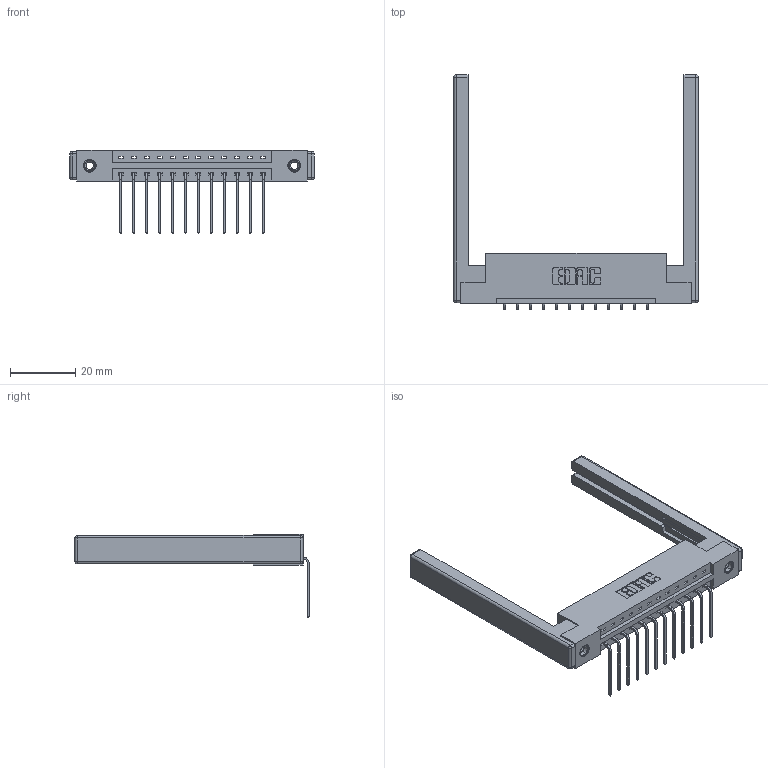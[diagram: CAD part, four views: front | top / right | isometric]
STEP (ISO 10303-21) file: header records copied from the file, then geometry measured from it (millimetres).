
FILE_DESCRIPTION (( 'STEP AP203' ), '1' );
FILE_NAME ('337-012-559-168.STEP', '2019-09-28T01:02:09', ( '' ), ( '' ), 'SwSTEP 2.0', 'SolidWorks 2016', '' );
FILE_SCHEMA (( 'CONFIG_CONTROL_DESIGN' ));
Length unit declared in the file: inch
Products named in the file (5): 345-250-001_345-250-001-102; 337 Part_Flush Mounting Lugs - 0.156 Dia-TI; 345-292-001_558 559 Tail - 1; 307-220-068; 337-012-559-168
Assembly tree (17 placements, depth 2):
  337-012-559-168
    337 Part_Flush Mounting Lugs - 0.156 Dia-TI
    345-292-001_558 559 Tail - 1  x12
    345-250-001_345-250-001-102  x2
    307-220-068  x2
Bounding box: 74.98 x 71.82 x 25.53 mm (x, y, z)
Volume: 11848.8 mm3; surface area: 11878.1 mm2
Topology: 17 solids, 17 shells, 1036 faces, 3029 edges, 1982 vertices
Faces by surface type: plane 734, cylinder 278, cone 12, sphere 8, torus 4
Entity records: 15644 total; most frequent: CARTESIAN_POINT 2679, ORIENTED_EDGE 2616, DIRECTION 2390, EDGE_CURVE 1308, LINE 1130, VECTOR 1130, VERTEX_POINT 862, AXIS2_PLACEMENT_3D 630
